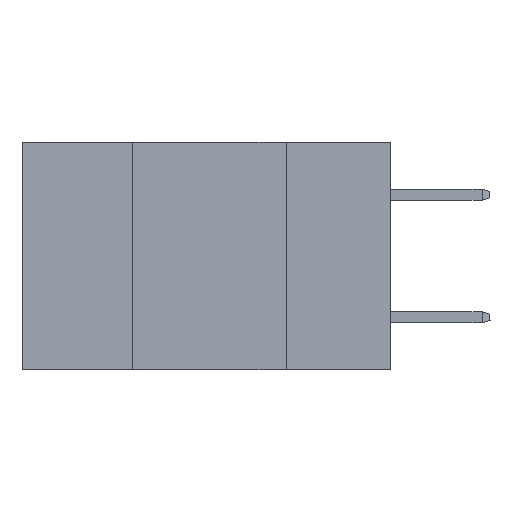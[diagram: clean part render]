
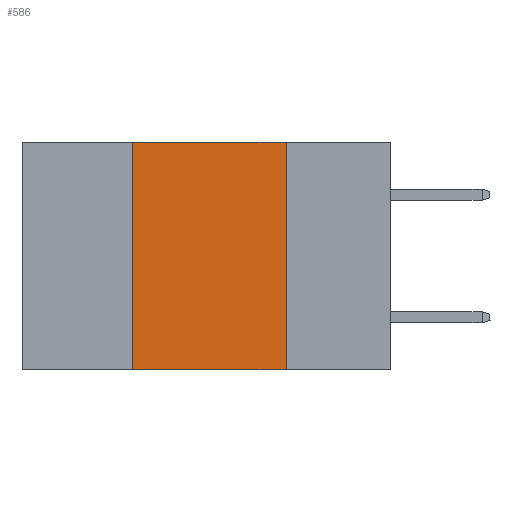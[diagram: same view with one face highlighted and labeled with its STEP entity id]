
A CAD part, left-side view. The second image highlights one B-rep face of the part: STEP entity #586.
In plain terms, the highlighted planar face has unit normal (-1, 0, 0).
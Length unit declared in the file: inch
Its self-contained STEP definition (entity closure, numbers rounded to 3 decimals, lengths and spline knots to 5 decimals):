
#475 = EDGE_CURVE ( 'NONE', #8918, #19886, #21896, .T. ) ;
#586 = ADVANCED_FACE ( 'NONE', ( #25038 ), #30019, .F. ) ;
#854 = CARTESIAN_POINT ( 'NONE',  ( 0., 0.42, 0. ) ) ;
#1126 = VECTOR ( 'NONE', #11806, 39.37008 ) ;
#1978 = DIRECTION ( 'NONE',  ( 0., 0., -1. ) ) ;
#2785 = VERTEX_POINT ( 'NONE', #3670 ) ;
#3059 = CARTESIAN_POINT ( 'NONE',  ( 0., 0.6, 0. ) ) ;
#3258 = DIRECTION ( 'NONE',  ( 1., 0., 0. ) ) ;
#3670 = CARTESIAN_POINT ( 'NONE',  ( 0., 0.17, -0.37 ) ) ;
#5080 = VECTOR ( 'NONE', #24729, 39.37008 ) ;
#6483 = ORIENTED_EDGE ( 'NONE', *, *, #475, .F. ) ;
#6811 = LINE ( 'NONE', #9060, #14543 ) ;
#7130 = CARTESIAN_POINT ( 'NONE',  ( 0., 0.6, -0.37 ) ) ;
#7901 = DIRECTION ( 'NONE',  ( 0., -1., 0. ) ) ;
#8918 = VERTEX_POINT ( 'NONE', #13852 ) ;
#9060 = CARTESIAN_POINT ( 'NONE',  ( 0., 0.17, 0. ) ) ;
#9253 = AXIS2_PLACEMENT_3D ( 'NONE', #15632, #3258, #13068 ) ;
#11806 = DIRECTION ( 'NONE',  ( 0., -1., 0. ) ) ;
#11834 = EDGE_LOOP ( 'NONE', ( #27918, #29724, #6483, #20272 ) ) ;
#12275 = LINE ( 'NONE', #7130, #1126 ) ;
#13068 = DIRECTION ( 'NONE',  ( 0., 0., -1. ) ) ;
#13852 = CARTESIAN_POINT ( 'NONE',  ( 0., 0.42, -0.37 ) ) ;
#14543 = VECTOR ( 'NONE', #1978, 39.37008 ) ;
#15632 = CARTESIAN_POINT ( 'NONE',  ( 0., 0.6, 0. ) ) ;
#17364 = LINE ( 'NONE', #3059, #25838 ) ;
#19804 = CARTESIAN_POINT ( 'NONE',  ( 0., 0.42, 0. ) ) ;
#19886 = VERTEX_POINT ( 'NONE', #854 ) ;
#20272 = ORIENTED_EDGE ( 'NONE', *, *, #27097, .T. ) ;
#21230 = CARTESIAN_POINT ( 'NONE',  ( 0., 0.17, 0. ) ) ;
#21330 = EDGE_CURVE ( 'NONE', #28976, #2785, #6811, .T. ) ;
#21896 = LINE ( 'NONE', #19804, #5080 ) ;
#22743 = EDGE_CURVE ( 'NONE', #19886, #28976, #17364, .T. ) ;
#24729 = DIRECTION ( 'NONE',  ( 0., 0., 1. ) ) ;
#25038 = FACE_OUTER_BOUND ( 'NONE', #11834, .T. ) ;
#25838 = VECTOR ( 'NONE', #7901, 39.37008 ) ;
#27097 = EDGE_CURVE ( 'NONE', #8918, #2785, #12275, .T. ) ;
#27918 = ORIENTED_EDGE ( 'NONE', *, *, #21330, .F. ) ;
#28976 = VERTEX_POINT ( 'NONE', #21230 ) ;
#29724 = ORIENTED_EDGE ( 'NONE', *, *, #22743, .F. ) ;
#30019 = PLANE ( 'NONE',  #9253 ) ;
